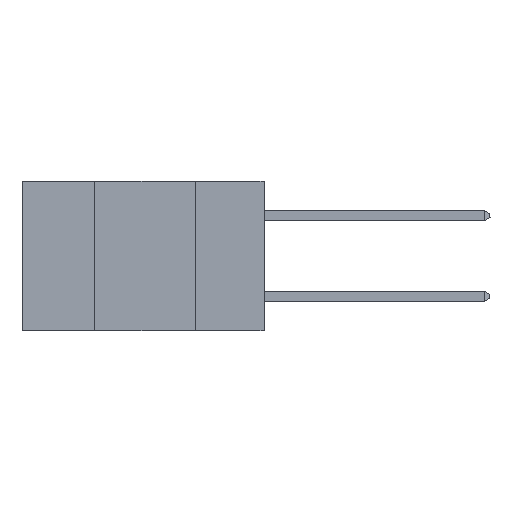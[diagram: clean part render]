
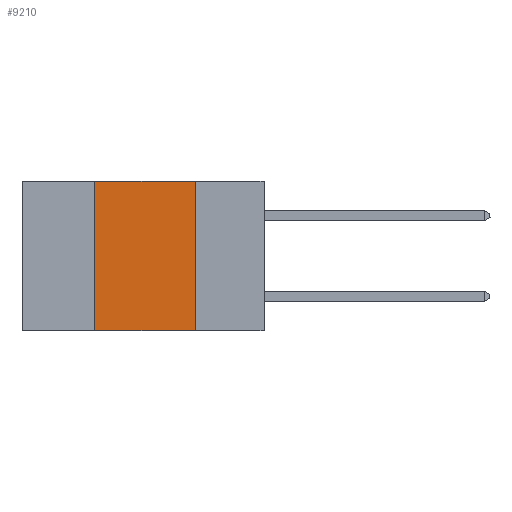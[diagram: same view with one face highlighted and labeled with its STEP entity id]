
A CAD part, left-side view. The second image highlights one B-rep face of the part: STEP entity #9210.
In plain terms, the highlighted planar face has unit normal (-1, 0, 0).
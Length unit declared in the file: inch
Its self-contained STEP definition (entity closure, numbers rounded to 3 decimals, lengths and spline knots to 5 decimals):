
#926 = EDGE_CURVE ( 'NONE', #9904, #11412, #14925, .T. ) ;
#1115 = DIRECTION ( 'NONE',  ( 1., 0., 0. ) ) ;
#1194 = LINE ( 'NONE', #14585, #3115 ) ;
#1211 = EDGE_CURVE ( 'NONE', #9904, #7963, #3735, .T. ) ;
#1631 = DIRECTION ( 'NONE',  ( 0., -1., 0. ) ) ;
#1958 = ORIENTED_EDGE ( 'NONE', *, *, #11613, .F. ) ;
#3115 = VECTOR ( 'NONE', #7101, 39.37008 ) ;
#3160 = EDGE_LOOP ( 'NONE', ( #6918, #1958, #3728, #11151 ) ) ;
#3211 = CARTESIAN_POINT ( 'NONE',  ( 0., 0.42, -0.37 ) ) ;
#3728 = ORIENTED_EDGE ( 'NONE', *, *, #926, .F. ) ;
#3735 = LINE ( 'NONE', #10149, #14354 ) ;
#3921 = DIRECTION ( 'NONE',  ( 0., 0., -1. ) ) ;
#4162 = VECTOR ( 'NONE', #15808, 39.37008 ) ;
#4398 = DIRECTION ( 'NONE',  ( 0., 0., 1. ) ) ;
#5306 = AXIS2_PLACEMENT_3D ( 'NONE', #13360, #1115, #3921 ) ;
#5999 = PLANE ( 'NONE',  #5306 ) ;
#6160 = CARTESIAN_POINT ( 'NONE',  ( 0., 0.17, -0.37 ) ) ;
#6302 = CARTESIAN_POINT ( 'NONE',  ( 0., 0.42, 0. ) ) ;
#6918 = ORIENTED_EDGE ( 'NONE', *, *, #13414, .F. ) ;
#7101 = DIRECTION ( 'NONE',  ( 0., -1., 0. ) ) ;
#7963 = VERTEX_POINT ( 'NONE', #6160 ) ;
#9210 = ADVANCED_FACE ( 'NONE', ( #13874 ), #5999, .F. ) ;
#9904 = VERTEX_POINT ( 'NONE', #3211 ) ;
#10149 = CARTESIAN_POINT ( 'NONE',  ( 0., 0.6, -0.37 ) ) ;
#11044 = VECTOR ( 'NONE', #4398, 39.37008 ) ;
#11151 = ORIENTED_EDGE ( 'NONE', *, *, #1211, .T. ) ;
#11412 = VERTEX_POINT ( 'NONE', #6302 ) ;
#11613 = EDGE_CURVE ( 'NONE', #11412, #12273, #1194, .T. ) ;
#11891 = LINE ( 'NONE', #14554, #4162 ) ;
#12273 = VERTEX_POINT ( 'NONE', #14922 ) ;
#12717 = CARTESIAN_POINT ( 'NONE',  ( 0., 0.42, 0. ) ) ;
#13360 = CARTESIAN_POINT ( 'NONE',  ( 0., 0.6, 0. ) ) ;
#13414 = EDGE_CURVE ( 'NONE', #12273, #7963, #11891, .T. ) ;
#13874 = FACE_OUTER_BOUND ( 'NONE', #3160, .T. ) ;
#14354 = VECTOR ( 'NONE', #1631, 39.37008 ) ;
#14554 = CARTESIAN_POINT ( 'NONE',  ( 0., 0.17, 0. ) ) ;
#14585 = CARTESIAN_POINT ( 'NONE',  ( 0., 0.6, 0. ) ) ;
#14922 = CARTESIAN_POINT ( 'NONE',  ( 0., 0.17, 0. ) ) ;
#14925 = LINE ( 'NONE', #12717, #11044 ) ;
#15808 = DIRECTION ( 'NONE',  ( 0., 0., -1. ) ) ;
